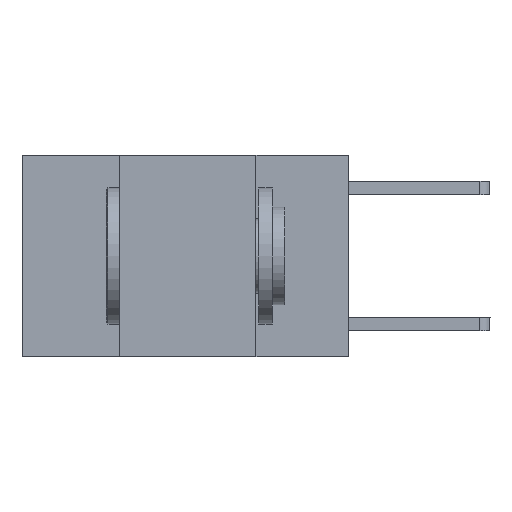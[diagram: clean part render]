
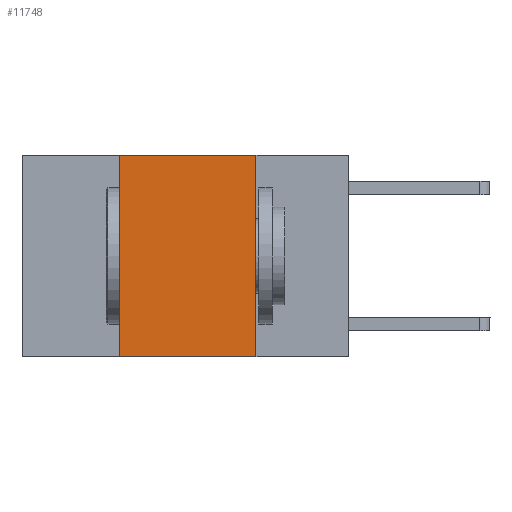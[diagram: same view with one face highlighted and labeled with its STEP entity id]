
A CAD part, left-side view. The second image highlights one B-rep face of the part: STEP entity #11748.
In plain terms, the highlighted planar face has unit normal (-1, 0, 0).
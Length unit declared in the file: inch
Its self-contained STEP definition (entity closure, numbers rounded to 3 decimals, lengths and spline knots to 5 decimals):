
#324 = VERTEX_POINT ( 'NONE', #10279 ) ;
#892 = CARTESIAN_POINT ( 'NONE',  ( 0., 0.17, 0. ) ) ;
#1129 = LINE ( 'NONE', #2078, #3329 ) ;
#1590 = CARTESIAN_POINT ( 'NONE',  ( 0., 0.42, 0. ) ) ;
#1633 = ORIENTED_EDGE ( 'NONE', *, *, #5459, .F. ) ;
#1719 = LINE ( 'NONE', #2211, #6352 ) ;
#2078 = CARTESIAN_POINT ( 'NONE',  ( 0., 0.6, -0.37 ) ) ;
#2211 = CARTESIAN_POINT ( 'NONE',  ( 0., 0.6, 0. ) ) ;
#2526 = ORIENTED_EDGE ( 'NONE', *, *, #3337, .T. ) ;
#3246 = EDGE_LOOP ( 'NONE', ( #6219, #10500, #1633, #2526 ) ) ;
#3329 = VECTOR ( 'NONE', #6748, 39.37008 ) ;
#3337 = EDGE_CURVE ( 'NONE', #7977, #7326, #1129, .T. ) ;
#3787 = EDGE_CURVE ( 'NONE', #6194, #7326, #10198, .T. ) ;
#4122 = PLANE ( 'NONE',  #9309 ) ;
#5018 = DIRECTION ( 'NONE',  ( 0., -1., 0. ) ) ;
#5023 = DIRECTION ( 'NONE',  ( 1., 0., 0. ) ) ;
#5459 = EDGE_CURVE ( 'NONE', #7977, #324, #7033, .T. ) ;
#5761 = DIRECTION ( 'NONE',  ( 0., 0., -1. ) ) ;
#5947 = FACE_OUTER_BOUND ( 'NONE', #3246, .T. ) ;
#6194 = VERTEX_POINT ( 'NONE', #892 ) ;
#6219 = ORIENTED_EDGE ( 'NONE', *, *, #3787, .F. ) ;
#6242 = DIRECTION ( 'NONE',  ( 0., 0., 1. ) ) ;
#6352 = VECTOR ( 'NONE', #5018, 39.37008 ) ;
#6435 = EDGE_CURVE ( 'NONE', #324, #6194, #1719, .T. ) ;
#6748 = DIRECTION ( 'NONE',  ( 0., -1., 0. ) ) ;
#7033 = LINE ( 'NONE', #1590, #9152 ) ;
#7178 = CARTESIAN_POINT ( 'NONE',  ( 0., 0.17, -0.37 ) ) ;
#7326 = VERTEX_POINT ( 'NONE', #7178 ) ;
#7977 = VERTEX_POINT ( 'NONE', #9943 ) ;
#9152 = VECTOR ( 'NONE', #6242, 39.37008 ) ;
#9309 = AXIS2_PLACEMENT_3D ( 'NONE', #10505, #5023, #11386 ) ;
#9943 = CARTESIAN_POINT ( 'NONE',  ( 0., 0.42, -0.37 ) ) ;
#10198 = LINE ( 'NONE', #11206, #10489 ) ;
#10279 = CARTESIAN_POINT ( 'NONE',  ( 0., 0.42, 0. ) ) ;
#10489 = VECTOR ( 'NONE', #5761, 39.37008 ) ;
#10500 = ORIENTED_EDGE ( 'NONE', *, *, #6435, .F. ) ;
#10505 = CARTESIAN_POINT ( 'NONE',  ( 0., 0.6, 0. ) ) ;
#11206 = CARTESIAN_POINT ( 'NONE',  ( 0., 0.17, 0. ) ) ;
#11386 = DIRECTION ( 'NONE',  ( 0., 0., -1. ) ) ;
#11748 = ADVANCED_FACE ( 'NONE', ( #5947 ), #4122, .F. ) ;
